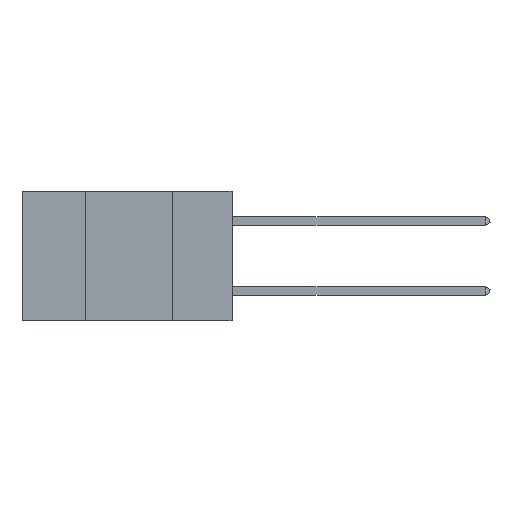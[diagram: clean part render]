
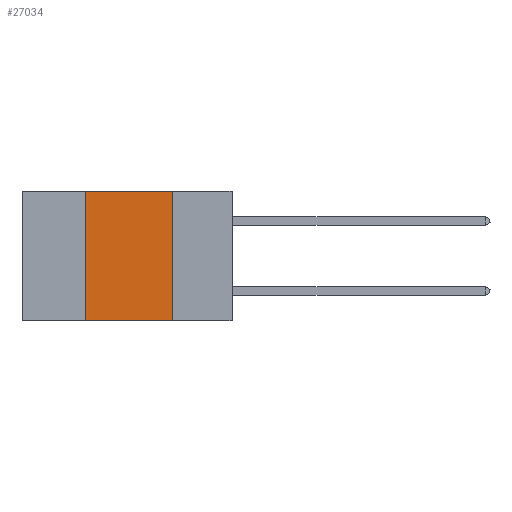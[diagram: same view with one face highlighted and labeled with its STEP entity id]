
A CAD part, left-side view. The second image highlights one B-rep face of the part: STEP entity #27034.
In plain terms, the highlighted planar face has unit normal (-1, 0, 0).
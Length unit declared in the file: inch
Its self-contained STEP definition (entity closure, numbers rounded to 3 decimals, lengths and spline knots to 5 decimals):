
#491 = VERTEX_POINT ( 'NONE', #22136 ) ;
#778 = VERTEX_POINT ( 'NONE', #39154 ) ;
#1499 = EDGE_CURVE ( 'NONE', #32733, #778, #11495, .T. ) ;
#2496 = CARTESIAN_POINT ( 'NONE',  ( 0., 0.42, 0. ) ) ;
#4328 = PLANE ( 'NONE',  #5552 ) ;
#5552 = AXIS2_PLACEMENT_3D ( 'NONE', #13690, #38051, #25440 ) ;
#5684 = ORIENTED_EDGE ( 'NONE', *, *, #38031, .F. ) ;
#7156 = VECTOR ( 'NONE', #16447, 39.37008 ) ;
#8104 = DIRECTION ( 'NONE',  ( 0., 0., 1. ) ) ;
#8278 = VERTEX_POINT ( 'NONE', #2496 ) ;
#10136 = CARTESIAN_POINT ( 'NONE',  ( 0., 0.6, -0.37 ) ) ;
#11440 = VECTOR ( 'NONE', #8104, 39.37008 ) ;
#11495 = LINE ( 'NONE', #10136, #7156 ) ;
#12023 = ORIENTED_EDGE ( 'NONE', *, *, #34295, .F. ) ;
#13690 = CARTESIAN_POINT ( 'NONE',  ( 0., 0.6, 0. ) ) ;
#16294 = CARTESIAN_POINT ( 'NONE',  ( 0., 0.42, 0. ) ) ;
#16447 = DIRECTION ( 'NONE',  ( 0., -1., 0. ) ) ;
#16688 = EDGE_LOOP ( 'NONE', ( #12023, #26662, #5684, #31436 ) ) ;
#18428 = VECTOR ( 'NONE', #33995, 39.37008 ) ;
#22053 = CARTESIAN_POINT ( 'NONE',  ( 0., 0.6, 0. ) ) ;
#22136 = CARTESIAN_POINT ( 'NONE',  ( 0., 0.17, 0. ) ) ;
#25440 = DIRECTION ( 'NONE',  ( 0., 0., -1. ) ) ;
#26582 = FACE_OUTER_BOUND ( 'NONE', #16688, .T. ) ;
#26662 = ORIENTED_EDGE ( 'NONE', *, *, #30283, .F. ) ;
#27034 = ADVANCED_FACE ( 'NONE', ( #26582 ), #4328, .F. ) ;
#27316 = VECTOR ( 'NONE', #37074, 39.37008 ) ;
#29445 = CARTESIAN_POINT ( 'NONE',  ( 0., 0.42, -0.37 ) ) ;
#30283 = EDGE_CURVE ( 'NONE', #8278, #491, #35408, .T. ) ;
#30928 = CARTESIAN_POINT ( 'NONE',  ( 0., 0.17, 0. ) ) ;
#31436 = ORIENTED_EDGE ( 'NONE', *, *, #1499, .T. ) ;
#32733 = VERTEX_POINT ( 'NONE', #29445 ) ;
#33995 = DIRECTION ( 'NONE',  ( 0., 0., -1. ) ) ;
#34295 = EDGE_CURVE ( 'NONE', #491, #778, #36016, .T. ) ;
#35408 = LINE ( 'NONE', #22053, #27316 ) ;
#36016 = LINE ( 'NONE', #30928, #18428 ) ;
#37074 = DIRECTION ( 'NONE',  ( 0., -1., 0. ) ) ;
#37187 = LINE ( 'NONE', #16294, #11440 ) ;
#38031 = EDGE_CURVE ( 'NONE', #32733, #8278, #37187, .T. ) ;
#38051 = DIRECTION ( 'NONE',  ( 1., 0., 0. ) ) ;
#39154 = CARTESIAN_POINT ( 'NONE',  ( 0., 0.17, -0.37 ) ) ;
